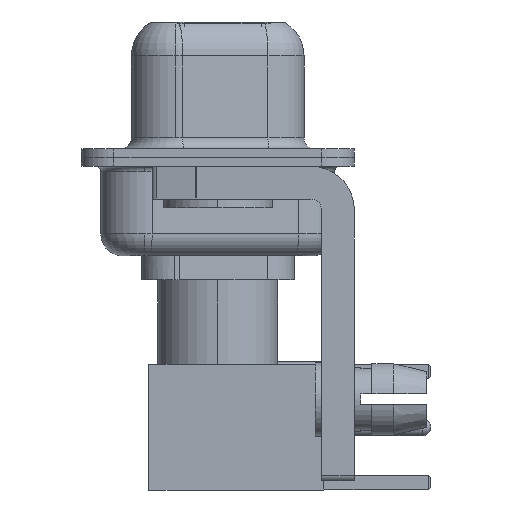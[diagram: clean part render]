
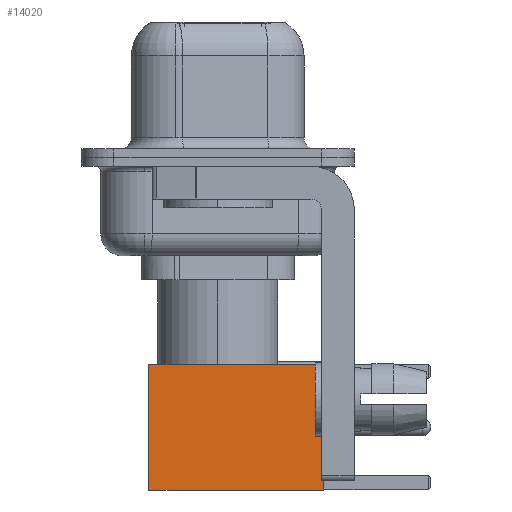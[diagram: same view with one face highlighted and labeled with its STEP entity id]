
A CAD part, left-side view. The second image highlights one B-rep face of the part: STEP entity #14020.
In plain terms, the highlighted face is planar.
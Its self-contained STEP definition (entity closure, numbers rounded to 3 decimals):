
#621 = VERTEX_POINT ( 'NONE', #19028 ) ;
#1263 = ORIENTED_EDGE ( 'NONE', *, *, #19520, .T. ) ;
#1363 = ORIENTED_EDGE ( 'NONE', *, *, #8461, .F. ) ;
#1742 = CARTESIAN_POINT ( 'NONE',  ( -2.875, 2.875, 0. ) ) ;
#2235 = DIRECTION ( 'NONE',  ( 0., 0., -1. ) ) ;
#2245 = VECTOR ( 'NONE', #2235, 1000. ) ;
#3630 = ORIENTED_EDGE ( 'NONE', *, *, #21183, .T. ) ;
#3895 = LINE ( 'NONE', #1742, #2245 ) ;
#4622 = CARTESIAN_POINT ( 'NONE',  ( 0., 2.875, 0. ) ) ;
#5114 = DIRECTION ( 'NONE',  ( 0., 1., 0. ) ) ;
#5263 = AXIS2_PLACEMENT_3D ( 'NONE', #7178, #5114, #11259 ) ;
#5360 = DIRECTION ( 'NONE',  ( -1., 0., 0. ) ) ;
#5402 = ORIENTED_EDGE ( 'NONE', *, *, #9299, .F. ) ;
#5619 = LINE ( 'NONE', #17597, #13688 ) ;
#7178 = CARTESIAN_POINT ( 'NONE',  ( 2.875, 2.875, 0. ) ) ;
#7334 = CARTESIAN_POINT ( 'NONE',  ( 2.875, 2.875, 0. ) ) ;
#7460 = DIRECTION ( 'NONE',  ( 0., 0., -1. ) ) ;
#8461 = EDGE_CURVE ( 'NONE', #8782, #12299, #3895, .T. ) ;
#8782 = VERTEX_POINT ( 'NONE', #12686 ) ;
#9117 = LINE ( 'NONE', #7334, #19248 ) ;
#9299 = EDGE_CURVE ( 'NONE', #621, #8782, #5619, .T. ) ;
#10067 = EDGE_LOOP ( 'NONE', ( #1263, #3630, #1363, #5402 ) ) ;
#11259 = DIRECTION ( 'NONE',  ( 0., 0., 1. ) ) ;
#11514 = VERTEX_POINT ( 'NONE', #12856 ) ;
#12299 = VERTEX_POINT ( 'NONE', #17943 ) ;
#12359 = VECTOR ( 'NONE', #12671, 1000. ) ;
#12671 = DIRECTION ( 'NONE',  ( -1., 0., 0. ) ) ;
#12686 = CARTESIAN_POINT ( 'NONE',  ( -2.875, 2.875, 8. ) ) ;
#12856 = CARTESIAN_POINT ( 'NONE',  ( 2.875, 2.875, 0. ) ) ;
#12927 = PLANE ( 'NONE',  #5263 ) ;
#13688 = VECTOR ( 'NONE', #5360, 1000. ) ;
#14020 = ADVANCED_FACE ( 'NONE', ( #22581 ), #12927, .T. ) ;
#17597 = CARTESIAN_POINT ( 'NONE',  ( 0., 2.875, 8. ) ) ;
#17943 = CARTESIAN_POINT ( 'NONE',  ( -2.875, 2.875, 0. ) ) ;
#19028 = CARTESIAN_POINT ( 'NONE',  ( 2.875, 2.875, 8. ) ) ;
#19248 = VECTOR ( 'NONE', #7460, 1000. ) ;
#19520 = EDGE_CURVE ( 'NONE', #621, #11514, #9117, .T. ) ;
#21183 = EDGE_CURVE ( 'NONE', #11514, #12299, #22078, .T. ) ;
#22078 = LINE ( 'NONE', #4622, #12359 ) ;
#22581 = FACE_OUTER_BOUND ( 'NONE', #10067, .T. ) ;
